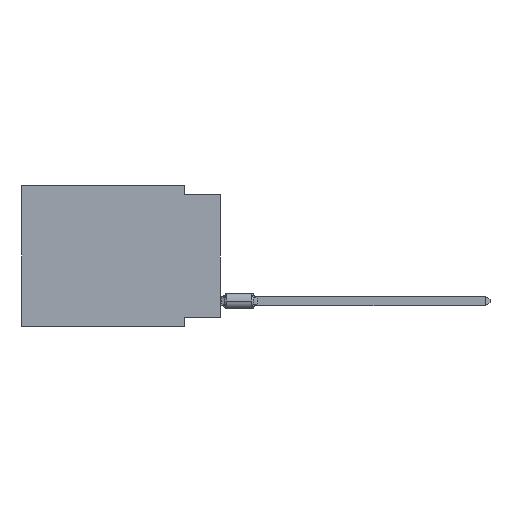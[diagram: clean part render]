
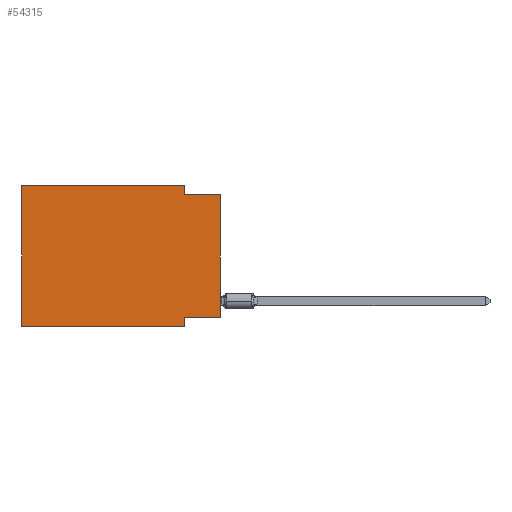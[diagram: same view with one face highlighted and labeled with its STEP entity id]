
A CAD part, left-side view. The second image highlights one B-rep face of the part: STEP entity #54315.
In plain terms, the highlighted planar face has unit normal (-1, 0, 0).
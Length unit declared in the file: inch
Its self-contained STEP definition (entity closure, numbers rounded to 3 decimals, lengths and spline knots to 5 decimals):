
#3113 = ORIENTED_EDGE ( 'NONE', *, *, #7801, .F. ) ;
#4182 = EDGE_CURVE ( 'NONE', #8275, #41287, #33694, .T. ) ;
#4243 = CARTESIAN_POINT ( 'NONE',  ( 0., 0., -0.365 ) ) ;
#7003 = LINE ( 'NONE', #27590, #49065 ) ;
#7801 = EDGE_CURVE ( 'NONE', #44659, #29287, #14764, .T. ) ;
#8275 = VERTEX_POINT ( 'NONE', #28225 ) ;
#8830 = VECTOR ( 'NONE', #35280, 39.37008 ) ;
#9266 = VECTOR ( 'NONE', #56667, 39.37008 ) ;
#10501 = EDGE_CURVE ( 'NONE', #8275, #29287, #66678, .T. ) ;
#11074 = CARTESIAN_POINT ( 'NONE',  ( 0., 0., -0.025 ) ) ;
#12327 = CARTESIAN_POINT ( 'NONE',  ( 0., 0.1, -0.025 ) ) ;
#12659 = CARTESIAN_POINT ( 'NONE',  ( 0., 0.55, 0. ) ) ;
#14558 = CARTESIAN_POINT ( 'NONE',  ( 0., 0., -0.365 ) ) ;
#14764 = LINE ( 'NONE', #26606, #40864 ) ;
#15266 = LINE ( 'NONE', #11074, #39471 ) ;
#15646 = VECTOR ( 'NONE', #19092, 39.37008 ) ;
#15732 = ORIENTED_EDGE ( 'NONE', *, *, #60517, .T. ) ;
#19092 = DIRECTION ( 'NONE',  ( 0., 1., 0. ) ) ;
#21243 = LINE ( 'NONE', #37276, #66945 ) ;
#21476 = LINE ( 'NONE', #32289, #30729 ) ;
#23865 = VERTEX_POINT ( 'NONE', #12327 ) ;
#26217 = EDGE_CURVE ( 'NONE', #41287, #62060, #7003, .T. ) ;
#26468 = EDGE_CURVE ( 'NONE', #62060, #23865, #21243, .T. ) ;
#26606 = CARTESIAN_POINT ( 'NONE',  ( 0., 0.1, -0.39 ) ) ;
#27590 = CARTESIAN_POINT ( 'NONE',  ( 0., 0.55, 0. ) ) ;
#28225 = CARTESIAN_POINT ( 'NONE',  ( 0., 0.55, -0.39 ) ) ;
#29019 = ORIENTED_EDGE ( 'NONE', *, *, #10501, .T. ) ;
#29287 = VERTEX_POINT ( 'NONE', #37222 ) ;
#29683 = CARTESIAN_POINT ( 'NONE',  ( 0., 0.55, 0. ) ) ;
#30729 = VECTOR ( 'NONE', #38534, 39.37008 ) ;
#31158 = DIRECTION ( 'NONE',  ( 0., 0., -1. ) ) ;
#32289 = CARTESIAN_POINT ( 'NONE',  ( 0., 0., 0. ) ) ;
#32296 = EDGE_LOOP ( 'NONE', ( #15732, #42829, #53659, #39306, #64342, #29019, #3113, #58274 ) ) ;
#33694 = LINE ( 'NONE', #55638, #9266 ) ;
#35213 = VERTEX_POINT ( 'NONE', #4243 ) ;
#35280 = DIRECTION ( 'NONE',  ( 0., -1., 0. ) ) ;
#35422 = CARTESIAN_POINT ( 'NONE',  ( 0., 0.1, 0. ) ) ;
#35634 = CARTESIAN_POINT ( 'NONE',  ( 0., 0.55, -0.39 ) ) ;
#36485 = CARTESIAN_POINT ( 'NONE',  ( 0., 0.1, -0.365 ) ) ;
#36960 = AXIS2_PLACEMENT_3D ( 'NONE', #29683, #61053, #50235 ) ;
#37209 = EDGE_CURVE ( 'NONE', #35213, #44659, #62311, .T. ) ;
#37222 = CARTESIAN_POINT ( 'NONE',  ( 0., 0.1, -0.39 ) ) ;
#37276 = CARTESIAN_POINT ( 'NONE',  ( 0., 0.1, 0. ) ) ;
#38534 = DIRECTION ( 'NONE',  ( 0., 0., 1. ) ) ;
#38728 = DIRECTION ( 'NONE',  ( 0., -1., 0. ) ) ;
#39306 = ORIENTED_EDGE ( 'NONE', *, *, #26217, .F. ) ;
#39471 = VECTOR ( 'NONE', #68265, 39.37008 ) ;
#40463 = FACE_OUTER_BOUND ( 'NONE', #32296, .T. ) ;
#40864 = VECTOR ( 'NONE', #31158, 39.37008 ) ;
#41287 = VERTEX_POINT ( 'NONE', #12659 ) ;
#42829 = ORIENTED_EDGE ( 'NONE', *, *, #67470, .F. ) ;
#43571 = CARTESIAN_POINT ( 'NONE',  ( 0., 0., -0.025 ) ) ;
#44659 = VERTEX_POINT ( 'NONE', #36485 ) ;
#49065 = VECTOR ( 'NONE', #38728, 39.37008 ) ;
#50235 = DIRECTION ( 'NONE',  ( 0., 0., -1. ) ) ;
#53659 = ORIENTED_EDGE ( 'NONE', *, *, #26468, .F. ) ;
#54315 = ADVANCED_FACE ( 'NONE', ( #40463 ), #66632, .F. ) ;
#55638 = CARTESIAN_POINT ( 'NONE',  ( 0., 0.55, 0. ) ) ;
#55839 = VERTEX_POINT ( 'NONE', #43571 ) ;
#56667 = DIRECTION ( 'NONE',  ( 0., 0., 1. ) ) ;
#58274 = ORIENTED_EDGE ( 'NONE', *, *, #37209, .F. ) ;
#58540 = DIRECTION ( 'NONE',  ( 0., 0., -1. ) ) ;
#60517 = EDGE_CURVE ( 'NONE', #35213, #55839, #21476, .T. ) ;
#61053 = DIRECTION ( 'NONE',  ( 1., 0., 0. ) ) ;
#62060 = VERTEX_POINT ( 'NONE', #35422 ) ;
#62311 = LINE ( 'NONE', #14558, #15646 ) ;
#64342 = ORIENTED_EDGE ( 'NONE', *, *, #4182, .F. ) ;
#66632 = PLANE ( 'NONE',  #36960 ) ;
#66678 = LINE ( 'NONE', #35634, #8830 ) ;
#66945 = VECTOR ( 'NONE', #58540, 39.37008 ) ;
#67470 = EDGE_CURVE ( 'NONE', #23865, #55839, #15266, .T. ) ;
#68265 = DIRECTION ( 'NONE',  ( 0., -1., 0. ) ) ;
